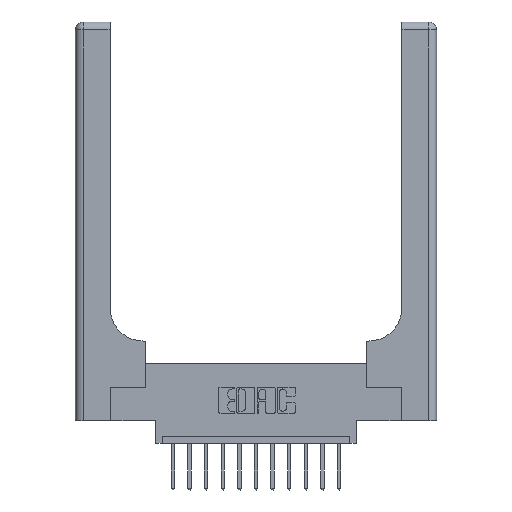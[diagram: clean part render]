
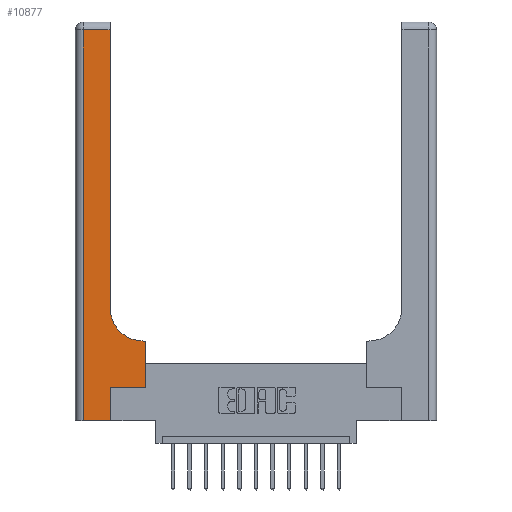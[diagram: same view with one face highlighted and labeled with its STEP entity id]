
A CAD part, top view. The second image highlights one B-rep face of the part: STEP entity #10877.
In plain terms, the highlighted planar face has unit normal (0, 0, 1).
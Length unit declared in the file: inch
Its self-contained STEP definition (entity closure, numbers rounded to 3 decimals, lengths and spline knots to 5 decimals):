
#206 = DIRECTION ( 'NONE',  ( -1., 0., 0. ) ) ;
#314 = LINE ( 'NONE', #14104, #14534 ) ;
#506 = ORIENTED_EDGE ( 'NONE', *, *, #9500, .T. ) ;
#580 = CARTESIAN_POINT ( 'NONE',  ( 0.06, 0., 0.37 ) ) ;
#840 = CARTESIAN_POINT ( 'NONE',  ( 0.51, 0.6, 0.37 ) ) ;
#1032 = VECTOR ( 'NONE', #9010, 39.37008 ) ;
#1116 = ORIENTED_EDGE ( 'NONE', *, *, #11032, .T. ) ;
#1235 = DIRECTION ( 'NONE',  ( 1., 0., 0. ) ) ;
#1320 = EDGE_CURVE ( 'NONE', #3176, #2827, #14484, .T. ) ;
#1480 = EDGE_CURVE ( 'NONE', #6672, #12561, #15440, .T. ) ;
#1481 = DIRECTION ( 'NONE',  ( 0., 0., -1. ) ) ;
#1683 = CARTESIAN_POINT ( 'NONE',  ( 0., 0., 0.37 ) ) ;
#1738 = LINE ( 'NONE', #1683, #2702 ) ;
#2702 = VECTOR ( 'NONE', #6853, 39.37008 ) ;
#2827 = VERTEX_POINT ( 'NONE', #10486 ) ;
#2839 = AXIS2_PLACEMENT_3D ( 'NONE', #13749, #16195, #9934 ) ;
#3082 = ORIENTED_EDGE ( 'NONE', *, *, #1320, .T. ) ;
#3176 = VERTEX_POINT ( 'NONE', #16272 ) ;
#3670 = LINE ( 'NONE', #15311, #14361 ) ;
#3764 = CARTESIAN_POINT ( 'NONE',  ( 0.51, 0.85, 0.37 ) ) ;
#3810 = ORIENTED_EDGE ( 'NONE', *, *, #5880, .T. ) ;
#3854 = CARTESIAN_POINT ( 'NONE',  ( 0.265, 0., 0.37 ) ) ;
#3897 = CARTESIAN_POINT ( 'NONE',  ( 0.265, 0., 0.37 ) ) ;
#4756 = LINE ( 'NONE', #3854, #1032 ) ;
#4938 = PLANE ( 'NONE',  #2839 ) ;
#4968 = CARTESIAN_POINT ( 'NONE',  ( 0., 2.94, 0.37 ) ) ;
#5230 = EDGE_CURVE ( 'NONE', #12726, #6266, #1738, .T. ) ;
#5880 = EDGE_CURVE ( 'NONE', #10506, #3176, #314, .T. ) ;
#6042 = ORIENTED_EDGE ( 'NONE', *, *, #7053, .T. ) ;
#6266 = VERTEX_POINT ( 'NONE', #3897 ) ;
#6672 = VERTEX_POINT ( 'NONE', #16064 ) ;
#6698 = VECTOR ( 'NONE', #12353, 39.37008 ) ;
#6775 = VECTOR ( 'NONE', #13008, 39.37008 ) ;
#6829 = EDGE_CURVE ( 'NONE', #11672, #10506, #8554, .T. ) ;
#6853 = DIRECTION ( 'NONE',  ( 1., 0., 0. ) ) ;
#6877 = CARTESIAN_POINT ( 'NONE',  ( 0.528, 0.25, 0.37 ) ) ;
#7053 = EDGE_CURVE ( 'NONE', #6266, #12283, #4756, .T. ) ;
#8155 = LINE ( 'NONE', #11512, #10296 ) ;
#8184 = EDGE_CURVE ( 'NONE', #12283, #6672, #8155, .T. ) ;
#8450 = CARTESIAN_POINT ( 'NONE',  ( 0.06, 3., 0.37 ) ) ;
#8554 = CIRCLE ( 'NONE', #11388, 0.25 ) ;
#8863 = CARTESIAN_POINT ( 'NONE',  ( 0.528, 0.6, 0.37 ) ) ;
#9010 = DIRECTION ( 'NONE',  ( 0., 1., 0. ) ) ;
#9500 = EDGE_CURVE ( 'NONE', #2827, #12726, #16127, .T. ) ;
#9855 = DIRECTION ( 'NONE',  ( -1., 0., 0. ) ) ;
#9934 = DIRECTION ( 'NONE',  ( -1., 0., 0. ) ) ;
#10296 = VECTOR ( 'NONE', #1235, 39.37008 ) ;
#10301 = DIRECTION ( 'NONE',  ( 1., 0., 0. ) ) ;
#10486 = CARTESIAN_POINT ( 'NONE',  ( 0.06, 2.94, 0.37 ) ) ;
#10506 = VERTEX_POINT ( 'NONE', #12878 ) ;
#10627 = FACE_OUTER_BOUND ( 'NONE', #13390, .T. ) ;
#10877 = ADVANCED_FACE ( 'NONE', ( #10627 ), #4938, .F. ) ;
#10911 = CARTESIAN_POINT ( 'NONE',  ( 0.265, 0.25, 0.37 ) ) ;
#11032 = EDGE_CURVE ( 'NONE', #12561, #11672, #3670, .T. ) ;
#11388 = AXIS2_PLACEMENT_3D ( 'NONE', #3764, #1481, #10301 ) ;
#11437 = ORIENTED_EDGE ( 'NONE', *, *, #5230, .T. ) ;
#11512 = CARTESIAN_POINT ( 'NONE',  ( 0.265, 0.25, 0.37 ) ) ;
#11672 = VERTEX_POINT ( 'NONE', #840 ) ;
#12200 = ORIENTED_EDGE ( 'NONE', *, *, #8184, .T. ) ;
#12283 = VERTEX_POINT ( 'NONE', #10911 ) ;
#12353 = DIRECTION ( 'NONE',  ( 0., -1., 0. ) ) ;
#12561 = VERTEX_POINT ( 'NONE', #8863 ) ;
#12726 = VERTEX_POINT ( 'NONE', #580 ) ;
#12789 = ORIENTED_EDGE ( 'NONE', *, *, #1480, .T. ) ;
#12878 = CARTESIAN_POINT ( 'NONE',  ( 0.26, 0.85, 0.37 ) ) ;
#13008 = DIRECTION ( 'NONE',  ( 0., 1., 0. ) ) ;
#13390 = EDGE_LOOP ( 'NONE', ( #3810, #3082, #506, #11437, #6042, #12200, #12789, #1116, #14569 ) ) ;
#13749 = CARTESIAN_POINT ( 'NONE',  ( 0., 3., 0.37 ) ) ;
#13884 = DIRECTION ( 'NONE',  ( 0., 1., 0. ) ) ;
#14096 = VECTOR ( 'NONE', #9855, 39.37008 ) ;
#14104 = CARTESIAN_POINT ( 'NONE',  ( 0.26, 3., 0.37 ) ) ;
#14361 = VECTOR ( 'NONE', #206, 39.37008 ) ;
#14484 = LINE ( 'NONE', #4968, #14096 ) ;
#14534 = VECTOR ( 'NONE', #13884, 39.37008 ) ;
#14569 = ORIENTED_EDGE ( 'NONE', *, *, #6829, .T. ) ;
#15311 = CARTESIAN_POINT ( 'NONE',  ( 0.26, 0.6, 0.37 ) ) ;
#15440 = LINE ( 'NONE', #6877, #6775 ) ;
#16064 = CARTESIAN_POINT ( 'NONE',  ( 0.528, 0.25, 0.37 ) ) ;
#16127 = LINE ( 'NONE', #8450, #6698 ) ;
#16195 = DIRECTION ( 'NONE',  ( 0., 0., -1. ) ) ;
#16272 = CARTESIAN_POINT ( 'NONE',  ( 0.26, 2.94, 0.37 ) ) ;
